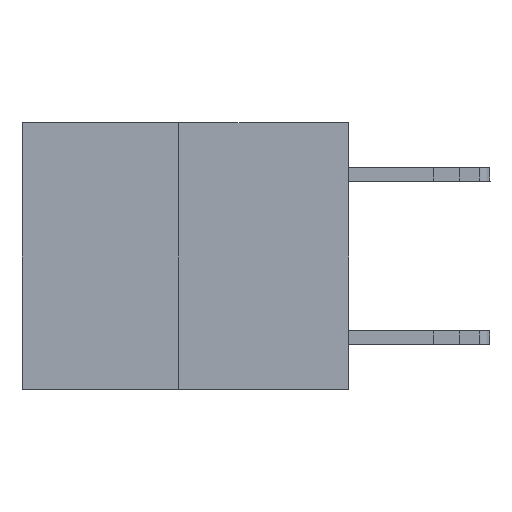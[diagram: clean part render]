
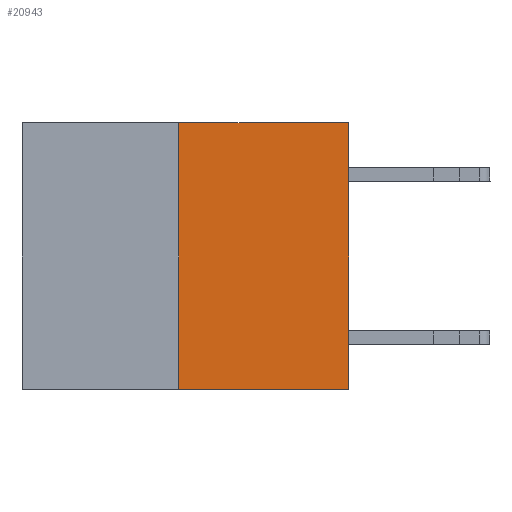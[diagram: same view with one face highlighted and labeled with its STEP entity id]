
A CAD part, left-side view. The second image highlights one B-rep face of the part: STEP entity #20943.
In plain terms, the highlighted planar face has unit normal (-1, 0, 0).
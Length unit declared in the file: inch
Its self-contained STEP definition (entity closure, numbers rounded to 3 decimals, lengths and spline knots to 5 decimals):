
#214 = CARTESIAN_POINT ( 'NONE',  ( 0., 0.6, 0. ) ) ;
#785 = ORIENTED_EDGE ( 'NONE', *, *, #2262, .F. ) ;
#1534 = LINE ( 'NONE', #21835, #23942 ) ;
#2262 = EDGE_CURVE ( 'NONE', #12104, #18775, #7990, .T. ) ;
#2978 = VERTEX_POINT ( 'NONE', #15193 ) ;
#3401 = CARTESIAN_POINT ( 'NONE',  ( 0., 0.6, 0. ) ) ;
#5695 = EDGE_CURVE ( 'NONE', #16175, #2978, #1534, .T. ) ;
#5856 = CARTESIAN_POINT ( 'NONE',  ( 0., 0.312, 0. ) ) ;
#5876 = EDGE_LOOP ( 'NONE', ( #18602, #18165, #15657, #785 ) ) ;
#7278 = PLANE ( 'NONE',  #18600 ) ;
#7990 = LINE ( 'NONE', #214, #14261 ) ;
#9916 = DIRECTION ( 'NONE',  ( 0., -1., 0. ) ) ;
#10399 = VECTOR ( 'NONE', #25669, 39.37008 ) ;
#10537 = EDGE_CURVE ( 'NONE', #2978, #18775, #20935, .T. ) ;
#11237 = DIRECTION ( 'NONE',  ( 0., 0., -1. ) ) ;
#12104 = VERTEX_POINT ( 'NONE', #5856 ) ;
#12468 = EDGE_CURVE ( 'NONE', #16175, #12104, #18921, .T. ) ;
#13940 = DIRECTION ( 'NONE',  ( 0., -1., 0. ) ) ;
#14261 = VECTOR ( 'NONE', #9916, 39.37008 ) ;
#15193 = CARTESIAN_POINT ( 'NONE',  ( 0., 0., -0.49 ) ) ;
#15263 = DIRECTION ( 'NONE',  ( 1., 0., 0. ) ) ;
#15657 = ORIENTED_EDGE ( 'NONE', *, *, #10537, .T. ) ;
#16175 = VERTEX_POINT ( 'NONE', #24638 ) ;
#18060 = CARTESIAN_POINT ( 'NONE',  ( 0., 0., 0. ) ) ;
#18165 = ORIENTED_EDGE ( 'NONE', *, *, #5695, .T. ) ;
#18400 = CARTESIAN_POINT ( 'NONE',  ( 0., 0., 0. ) ) ;
#18600 = AXIS2_PLACEMENT_3D ( 'NONE', #3401, #15263, #11237 ) ;
#18602 = ORIENTED_EDGE ( 'NONE', *, *, #12468, .F. ) ;
#18775 = VERTEX_POINT ( 'NONE', #18400 ) ;
#18921 = LINE ( 'NONE', #23678, #10399 ) ;
#20137 = DIRECTION ( 'NONE',  ( 0., 0., 1. ) ) ;
#20935 = LINE ( 'NONE', #18060, #25973 ) ;
#20943 = ADVANCED_FACE ( 'NONE', ( #25619 ), #7278, .F. ) ;
#21835 = CARTESIAN_POINT ( 'NONE',  ( 0., 0.6, -0.49 ) ) ;
#23678 = CARTESIAN_POINT ( 'NONE',  ( 0., 0.312, -0.49 ) ) ;
#23942 = VECTOR ( 'NONE', #13940, 39.37008 ) ;
#24638 = CARTESIAN_POINT ( 'NONE',  ( 0., 0.312, -0.49 ) ) ;
#25619 = FACE_OUTER_BOUND ( 'NONE', #5876, .T. ) ;
#25669 = DIRECTION ( 'NONE',  ( 0., 0., 1. ) ) ;
#25973 = VECTOR ( 'NONE', #20137, 39.37008 ) ;
